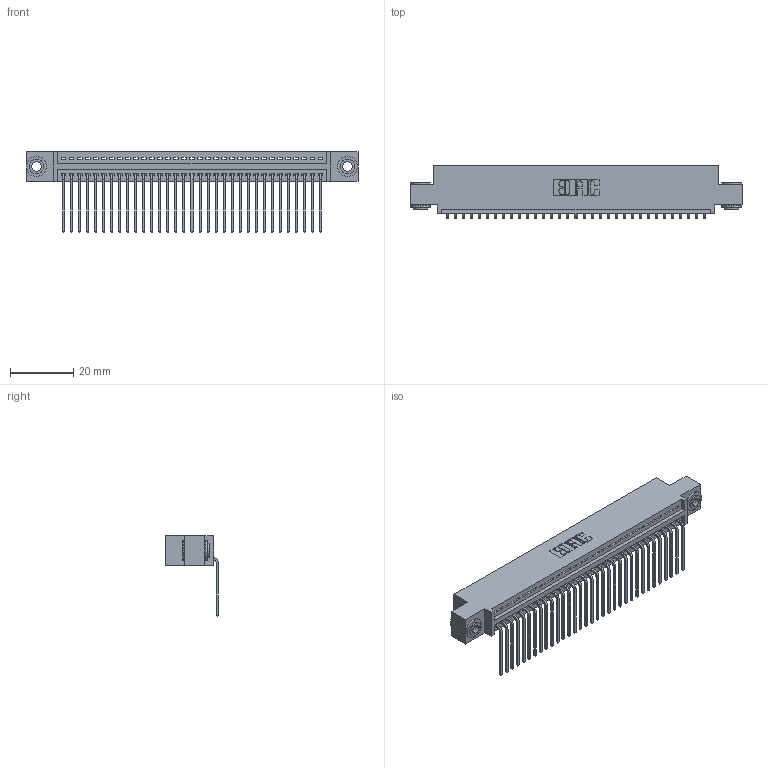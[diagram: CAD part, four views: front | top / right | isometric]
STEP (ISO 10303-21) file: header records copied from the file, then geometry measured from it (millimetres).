
FILE_DESCRIPTION (( 'STEP AP203' ), '1' );
FILE_NAME ('345-033-559-403.STEP', '2018-08-28T23:16:23', ( '' ), ( '' ), 'SwSTEP 2.0', 'SolidWorks 2016', '' );
FILE_SCHEMA (( 'CONFIG_CONTROL_DESIGN' ));
Length unit declared in the file: inch
Products named in the file (4): 345-250-002_345-250-002-102; 345-033-559-403; 345 Part_0.110 Offset - 0.156 Dia-TH; 345-292-001_558 559 Tail - 1
Assembly tree (36 placements, depth 2):
  345-033-559-403
    345 Part_0.110 Offset - 0.156 Dia-TH
    345-292-001_558 559 Tail - 1  x33
    345-250-002_345-250-002-102  x2
Bounding box: 105.03 x 16.75 x 25.53 mm (x, y, z)
Volume: 9958 mm3; surface area: 14053.4 mm2
Topology: 36 solids, 36 shells, 2148 faces, 6435 edges, 4242 vertices
Faces by surface type: plane 1480, cylinder 660, cone 8
Entity records: 26914 total; most frequent: CARTESIAN_POINT 4642, ORIENTED_EDGE 4602, DIRECTION 4097, EDGE_CURVE 2301, VECTOR 2013, LINE 2013, VERTEX_POINT 1530, AXIS2_PLACEMENT_3D 1042
